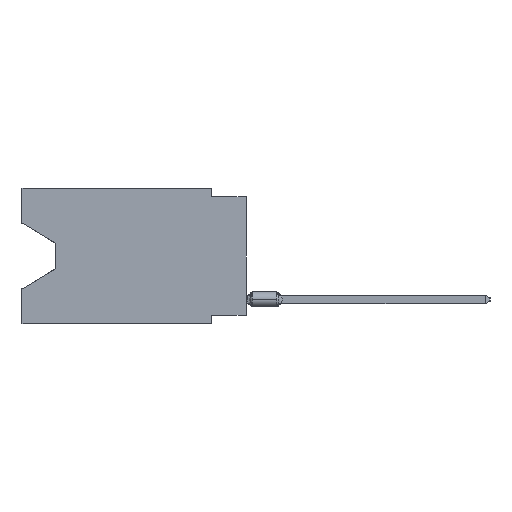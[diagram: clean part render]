
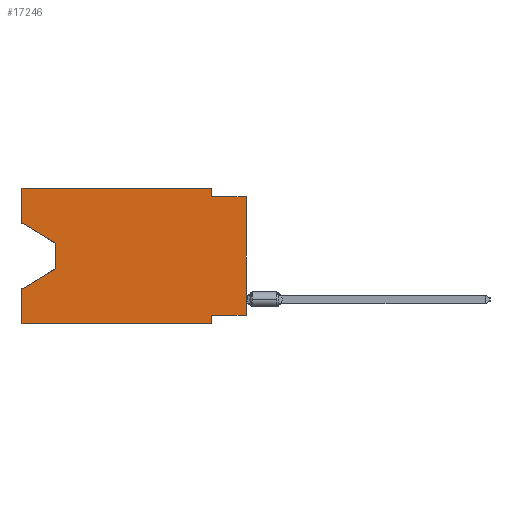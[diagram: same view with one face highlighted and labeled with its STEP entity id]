
A CAD part, left-side view. The second image highlights one B-rep face of the part: STEP entity #17246.
In plain terms, the highlighted planar face has unit normal (-1, 0, 0).
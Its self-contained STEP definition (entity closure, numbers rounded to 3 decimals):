
#111 = VECTOR ( 'NONE', #44921, 1000. ) ;
#208 = CARTESIAN_POINT ( 'NONE',  ( 0., 13.97, -4.013 ) ) ;
#845 = VERTEX_POINT ( 'NONE', #1688 ) ;
#1496 = ORIENTED_EDGE ( 'NONE', *, *, #43372, .T. ) ;
#1579 = ORIENTED_EDGE ( 'NONE', *, *, #6669, .F. ) ;
#1595 = LINE ( 'NONE', #29798, #35884 ) ;
#1688 = CARTESIAN_POINT ( 'NONE',  ( 0., 16.383, -7.36 ) ) ;
#1788 = CARTESIAN_POINT ( 'NONE',  ( 0., 2.54, -0.635 ) ) ;
#2097 = DIRECTION ( 'NONE',  ( 0., -1., 0. ) ) ;
#2161 = VECTOR ( 'NONE', #6901, 1000. ) ;
#2401 = ORIENTED_EDGE ( 'NONE', *, *, #33328, .T. ) ;
#2488 = VECTOR ( 'NONE', #7537, 1000. ) ;
#2827 = CARTESIAN_POINT ( 'NONE',  ( 0., 16.383, -9.906 ) ) ;
#3222 = LINE ( 'NONE', #21458, #8121 ) ;
#5020 = CARTESIAN_POINT ( 'NONE',  ( 0., 2.54, -9.906 ) ) ;
#5705 = EDGE_CURVE ( 'NONE', #29817, #5954, #26013, .T. ) ;
#5954 = VERTEX_POINT ( 'NONE', #6344 ) ;
#6071 = VERTEX_POINT ( 'NONE', #7712 ) ;
#6335 = VERTEX_POINT ( 'NONE', #20364 ) ;
#6344 = CARTESIAN_POINT ( 'NONE',  ( 0., 13.97, -5.893 ) ) ;
#6624 = AXIS2_PLACEMENT_3D ( 'NONE', #24761, #28233, #35182 ) ;
#6669 = EDGE_CURVE ( 'NONE', #31190, #33853, #42138, .T. ) ;
#6833 = CARTESIAN_POINT ( 'NONE',  ( 0., 2.54, -9.271 ) ) ;
#6901 = DIRECTION ( 'NONE',  ( 0., 0., 1. ) ) ;
#7537 = DIRECTION ( 'NONE',  ( 0., 0., -1. ) ) ;
#7712 = CARTESIAN_POINT ( 'NONE',  ( 0., 2.54, -9.906 ) ) ;
#8121 = VECTOR ( 'NONE', #20995, 1000. ) ;
#8293 = DIRECTION ( 'NONE',  ( 0., 0., 1. ) ) ;
#8332 = VECTOR ( 'NONE', #34054, 1000. ) ;
#8660 = EDGE_CURVE ( 'NONE', #25630, #45383, #41737, .T. ) ;
#8666 = DIRECTION ( 'NONE',  ( 0., 0.855, -0.519 ) ) ;
#9006 = DIRECTION ( 'NONE',  ( 0., -1., 0. ) ) ;
#9822 = CARTESIAN_POINT ( 'NONE',  ( 0., 16.383, -2.546 ) ) ;
#10034 = DIRECTION ( 'NONE',  ( 0., -0.855, -0.519 ) ) ;
#10066 = EDGE_CURVE ( 'NONE', #38206, #845, #10359, .T. ) ;
#10359 = LINE ( 'NONE', #38566, #2161 ) ;
#11844 = EDGE_CURVE ( 'NONE', #33853, #6071, #40608, .T. ) ;
#12586 = VECTOR ( 'NONE', #33010, 1000. ) ;
#12665 = CARTESIAN_POINT ( 'NONE',  ( 0., 2.54, 0. ) ) ;
#12786 = CARTESIAN_POINT ( 'NONE',  ( 0., 0., -0.635 ) ) ;
#12927 = LINE ( 'NONE', #30273, #31346 ) ;
#13503 = CARTESIAN_POINT ( 'NONE',  ( 0., 0., -9.271 ) ) ;
#14113 = CARTESIAN_POINT ( 'NONE',  ( 0., 0., -9.271 ) ) ;
#17246 = ADVANCED_FACE ( 'NONE', ( #23847 ), #37976, .F. ) ;
#17483 = EDGE_CURVE ( 'NONE', #6335, #25630, #40023, .T. ) ;
#17804 = EDGE_LOOP ( 'NONE', ( #1496, #24014, #39794, #44418, #2401, #23276, #1579, #26619, #28621, #38398, #35805, #37622 ) ) ;
#19291 = CARTESIAN_POINT ( 'NONE',  ( 0., 13.97, -5.893 ) ) ;
#19644 = CARTESIAN_POINT ( 'NONE',  ( 0., 16.383, 0. ) ) ;
#20364 = CARTESIAN_POINT ( 'NONE',  ( 0., 16.383, 0. ) ) ;
#20445 = CARTESIAN_POINT ( 'NONE',  ( 0., 2.54, 0. ) ) ;
#20937 = EDGE_CURVE ( 'NONE', #33586, #6335, #3222, .T. ) ;
#20995 = DIRECTION ( 'NONE',  ( 0., 0., 1. ) ) ;
#21458 = CARTESIAN_POINT ( 'NONE',  ( 0., 16.383, 0. ) ) ;
#22121 = CARTESIAN_POINT ( 'NONE',  ( 0., 16.383, -2.546 ) ) ;
#23054 = EDGE_CURVE ( 'NONE', #31190, #44477, #1595, .T. ) ;
#23276 = ORIENTED_EDGE ( 'NONE', *, *, #11844, .F. ) ;
#23847 = FACE_OUTER_BOUND ( 'NONE', #17804, .T. ) ;
#24014 = ORIENTED_EDGE ( 'NONE', *, *, #5705, .T. ) ;
#24761 = CARTESIAN_POINT ( 'NONE',  ( 0., 16.383, 0. ) ) ;
#25105 = CARTESIAN_POINT ( 'NONE',  ( 0., 13.97, -4.013 ) ) ;
#25630 = VERTEX_POINT ( 'NONE', #12665 ) ;
#26013 = LINE ( 'NONE', #25105, #2488 ) ;
#26533 = VECTOR ( 'NONE', #10034, 1000. ) ;
#26619 = ORIENTED_EDGE ( 'NONE', *, *, #23054, .T. ) ;
#28233 = DIRECTION ( 'NONE',  ( 1., 0., 0. ) ) ;
#28286 = EDGE_CURVE ( 'NONE', #5954, #845, #44012, .T. ) ;
#28621 = ORIENTED_EDGE ( 'NONE', *, *, #40228, .F. ) ;
#29798 = CARTESIAN_POINT ( 'NONE',  ( 0., 0., 0. ) ) ;
#29817 = VERTEX_POINT ( 'NONE', #208 ) ;
#30273 = CARTESIAN_POINT ( 'NONE',  ( 0., 16.383, -9.906 ) ) ;
#31190 = VERTEX_POINT ( 'NONE', #14113 ) ;
#31346 = VECTOR ( 'NONE', #9006, 1000. ) ;
#31707 = VECTOR ( 'NONE', #2097, 1000. ) ;
#33010 = DIRECTION ( 'NONE',  ( 0., 0., -1. ) ) ;
#33328 = EDGE_CURVE ( 'NONE', #38206, #6071, #12927, .T. ) ;
#33586 = VERTEX_POINT ( 'NONE', #22121 ) ;
#33853 = VERTEX_POINT ( 'NONE', #6833 ) ;
#34054 = DIRECTION ( 'NONE',  ( 0., -1., 0. ) ) ;
#35182 = DIRECTION ( 'NONE',  ( 0., 0., -1. ) ) ;
#35805 = ORIENTED_EDGE ( 'NONE', *, *, #17483, .F. ) ;
#35884 = VECTOR ( 'NONE', #8293, 1000. ) ;
#36123 = CARTESIAN_POINT ( 'NONE',  ( 0., 0., -0.635 ) ) ;
#37622 = ORIENTED_EDGE ( 'NONE', *, *, #20937, .F. ) ;
#37976 = PLANE ( 'NONE',  #6624 ) ;
#37983 = LINE ( 'NONE', #12786, #8332 ) ;
#38206 = VERTEX_POINT ( 'NONE', #2827 ) ;
#38266 = DIRECTION ( 'NONE',  ( 0., 0., -1. ) ) ;
#38398 = ORIENTED_EDGE ( 'NONE', *, *, #8660, .F. ) ;
#38566 = CARTESIAN_POINT ( 'NONE',  ( 0., 16.383, 0. ) ) ;
#39794 = ORIENTED_EDGE ( 'NONE', *, *, #28286, .T. ) ;
#40023 = LINE ( 'NONE', #19644, #31707 ) ;
#40228 = EDGE_CURVE ( 'NONE', #45383, #44477, #37983, .T. ) ;
#40608 = LINE ( 'NONE', #5020, #12586 ) ;
#40716 = VECTOR ( 'NONE', #8666, 1000. ) ;
#41715 = LINE ( 'NONE', #9822, #26533 ) ;
#41737 = LINE ( 'NONE', #20445, #43832 ) ;
#42138 = LINE ( 'NONE', #13503, #111 ) ;
#43372 = EDGE_CURVE ( 'NONE', #33586, #29817, #41715, .T. ) ;
#43832 = VECTOR ( 'NONE', #38266, 1000. ) ;
#44012 = LINE ( 'NONE', #19291, #40716 ) ;
#44418 = ORIENTED_EDGE ( 'NONE', *, *, #10066, .F. ) ;
#44477 = VERTEX_POINT ( 'NONE', #36123 ) ;
#44921 = DIRECTION ( 'NONE',  ( 0., 1., 0. ) ) ;
#45383 = VERTEX_POINT ( 'NONE', #1788 ) ;
